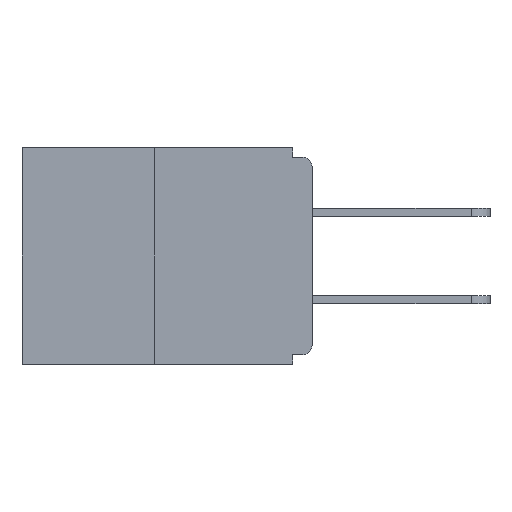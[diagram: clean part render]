
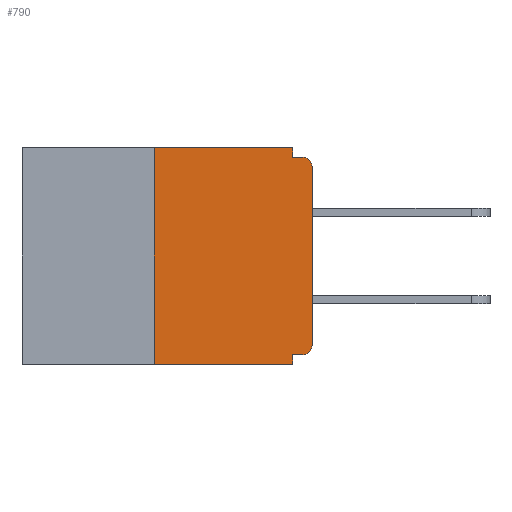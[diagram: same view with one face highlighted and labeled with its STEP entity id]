
A CAD part, left-side view. The second image highlights one B-rep face of the part: STEP entity #790.
In plain terms, the highlighted planar face has unit normal (-1, 0, 0).
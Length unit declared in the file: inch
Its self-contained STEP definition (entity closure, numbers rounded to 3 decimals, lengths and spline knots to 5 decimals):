
#377 = CARTESIAN_POINT ( 'NONE',  ( 0., 0.015, -0.03 ) ) ;
#415 = CARTESIAN_POINT ( 'NONE',  ( 0., 0.031, -0.015 ) ) ;
#677 = CARTESIAN_POINT ( 'NONE',  ( 0., 0.031, -0.343 ) ) ;
#790 = ADVANCED_FACE ( 'NONE', ( #816 ), #13683, .F. ) ;
#816 = FACE_OUTER_BOUND ( 'NONE', #12229, .T. ) ;
#969 = VERTEX_POINT ( 'NONE', #677 ) ;
#1039 = VECTOR ( 'NONE', #13028, 39.37008 ) ;
#1089 = VERTEX_POINT ( 'NONE', #8717 ) ;
#1174 = CARTESIAN_POINT ( 'NONE',  ( 0., 0.46, 0. ) ) ;
#1215 = DIRECTION ( 'NONE',  ( 0., 0., 1. ) ) ;
#1245 = EDGE_CURVE ( 'NONE', #1089, #2468, #14351, .T. ) ;
#1248 = VECTOR ( 'NONE', #9305, 39.37008 ) ;
#1377 = DIRECTION ( 'NONE',  ( 0., 1., 0. ) ) ;
#1516 = LINE ( 'NONE', #5505, #9867 ) ;
#2017 = CIRCLE ( 'NONE', #11576, 0.015 ) ;
#2221 = VERTEX_POINT ( 'NONE', #7350 ) ;
#2223 = CARTESIAN_POINT ( 'NONE',  ( 0., 0.031, -0.343 ) ) ;
#2466 = EDGE_CURVE ( 'NONE', #2221, #1089, #2017, .T. ) ;
#2468 = VERTEX_POINT ( 'NONE', #13284 ) ;
#2556 = ORIENTED_EDGE ( 'NONE', *, *, #12394, .F. ) ;
#2902 = ORIENTED_EDGE ( 'NONE', *, *, #5650, .F. ) ;
#3270 = ORIENTED_EDGE ( 'NONE', *, *, #10298, .T. ) ;
#3366 = LINE ( 'NONE', #7875, #5875 ) ;
#3400 = CARTESIAN_POINT ( 'NONE',  ( 0., 0., 0. ) ) ;
#3451 = VECTOR ( 'NONE', #1377, 39.37008 ) ;
#3470 = VECTOR ( 'NONE', #1215, 39.37008 ) ;
#3504 = VERTEX_POINT ( 'NONE', #415 ) ;
#4183 = CARTESIAN_POINT ( 'NONE',  ( 0., 0.015, -0.313 ) ) ;
#4440 = CARTESIAN_POINT ( 'NONE',  ( 0., 0.031, 0. ) ) ;
#4517 = LINE ( 'NONE', #2223, #11091 ) ;
#4660 = EDGE_CURVE ( 'NONE', #8889, #12181, #5185, .T. ) ;
#4957 = CARTESIAN_POINT ( 'NONE',  ( 0., 0.25, 0. ) ) ;
#5185 = LINE ( 'NONE', #13832, #1248 ) ;
#5505 = CARTESIAN_POINT ( 'NONE',  ( 0., 0.031, 0. ) ) ;
#5650 = EDGE_CURVE ( 'NONE', #8825, #8889, #9434, .T. ) ;
#5695 = CARTESIAN_POINT ( 'NONE',  ( 0., 0.015, -0.015 ) ) ;
#5875 = VECTOR ( 'NONE', #6667, 39.37008 ) ;
#6268 = DIRECTION ( 'NONE',  ( -1., 0., 0. ) ) ;
#6543 = DIRECTION ( 'NONE',  ( 0., -1., 0. ) ) ;
#6593 = CARTESIAN_POINT ( 'NONE',  ( 0., 0.46, -0.343 ) ) ;
#6667 = DIRECTION ( 'NONE',  ( 0., -1., 0. ) ) ;
#6841 = DIRECTION ( 'NONE',  ( 0., 0., -1. ) ) ;
#7291 = EDGE_CURVE ( 'NONE', #8825, #969, #12963, .T. ) ;
#7316 = LINE ( 'NONE', #9311, #3451 ) ;
#7350 = CARTESIAN_POINT ( 'NONE',  ( 0., 0.015, -0.328 ) ) ;
#7576 = AXIS2_PLACEMENT_3D ( 'NONE', #377, #6268, #10635 ) ;
#7875 = CARTESIAN_POINT ( 'NONE',  ( 0., 0., -0.015 ) ) ;
#8072 = DIRECTION ( 'NONE',  ( 1., 0., 0. ) ) ;
#8717 = CARTESIAN_POINT ( 'NONE',  ( 0., 0., -0.313 ) ) ;
#8722 = ORIENTED_EDGE ( 'NONE', *, *, #7291, .T. ) ;
#8825 = VERTEX_POINT ( 'NONE', #8849 ) ;
#8849 = CARTESIAN_POINT ( 'NONE',  ( 0., 0.25, -0.343 ) ) ;
#8889 = VERTEX_POINT ( 'NONE', #10050 ) ;
#8921 = EDGE_CURVE ( 'NONE', #12181, #3504, #1516, .T. ) ;
#9045 = ORIENTED_EDGE ( 'NONE', *, *, #12245, .F. ) ;
#9060 = DIRECTION ( 'NONE',  ( 0., 0., -1. ) ) ;
#9128 = ORIENTED_EDGE ( 'NONE', *, *, #10434, .F. ) ;
#9305 = DIRECTION ( 'NONE',  ( 0., -1., 0. ) ) ;
#9311 = CARTESIAN_POINT ( 'NONE',  ( 0., 0., -0.328 ) ) ;
#9418 = VECTOR ( 'NONE', #6543, 39.37008 ) ;
#9434 = LINE ( 'NONE', #4957, #1039 ) ;
#9744 = ORIENTED_EDGE ( 'NONE', *, *, #8921, .F. ) ;
#9867 = VECTOR ( 'NONE', #11297, 39.37008 ) ;
#10050 = CARTESIAN_POINT ( 'NONE',  ( 0., 0.25, 0. ) ) ;
#10190 = ORIENTED_EDGE ( 'NONE', *, *, #2466, .T. ) ;
#10298 = EDGE_CURVE ( 'NONE', #2468, #13721, #10910, .T. ) ;
#10434 = EDGE_CURVE ( 'NONE', #10659, #969, #4517, .T. ) ;
#10635 = DIRECTION ( 'NONE',  ( 0., 0., -1. ) ) ;
#10659 = VERTEX_POINT ( 'NONE', #10799 ) ;
#10799 = CARTESIAN_POINT ( 'NONE',  ( 0., 0.031, -0.328 ) ) ;
#10910 = CIRCLE ( 'NONE', #7576, 0.015 ) ;
#11091 = VECTOR ( 'NONE', #6841, 39.37008 ) ;
#11297 = DIRECTION ( 'NONE',  ( 0., 0., -1. ) ) ;
#11576 = AXIS2_PLACEMENT_3D ( 'NONE', #4183, #12265, #14534 ) ;
#12181 = VERTEX_POINT ( 'NONE', #4440 ) ;
#12229 = EDGE_LOOP ( 'NONE', ( #12395, #2902, #8722, #9128, #2556, #10190, #13978, #3270, #9045, #9744 ) ) ;
#12245 = EDGE_CURVE ( 'NONE', #3504, #13721, #3366, .T. ) ;
#12265 = DIRECTION ( 'NONE',  ( -1., 0., 0. ) ) ;
#12394 = EDGE_CURVE ( 'NONE', #2221, #10659, #7316, .T. ) ;
#12395 = ORIENTED_EDGE ( 'NONE', *, *, #4660, .F. ) ;
#12963 = LINE ( 'NONE', #6593, #9418 ) ;
#12993 = AXIS2_PLACEMENT_3D ( 'NONE', #1174, #8072, #9060 ) ;
#13028 = DIRECTION ( 'NONE',  ( 0., 0., 1. ) ) ;
#13284 = CARTESIAN_POINT ( 'NONE',  ( 0., 0., -0.03 ) ) ;
#13683 = PLANE ( 'NONE',  #12993 ) ;
#13721 = VERTEX_POINT ( 'NONE', #5695 ) ;
#13832 = CARTESIAN_POINT ( 'NONE',  ( 0., 0.46, 0. ) ) ;
#13978 = ORIENTED_EDGE ( 'NONE', *, *, #1245, .T. ) ;
#14351 = LINE ( 'NONE', #3400, #3470 ) ;
#14534 = DIRECTION ( 'NONE',  ( 0., 0., -1. ) ) ;
